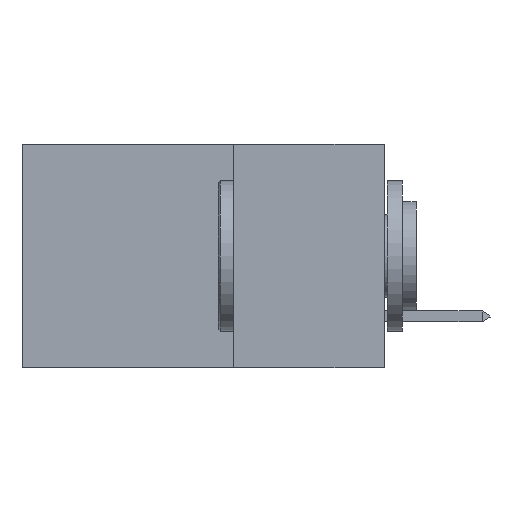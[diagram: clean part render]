
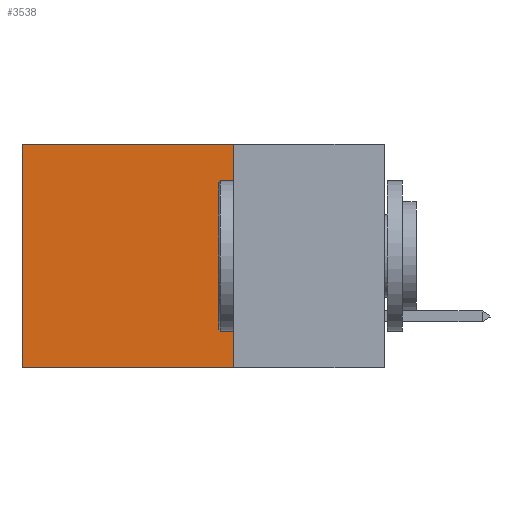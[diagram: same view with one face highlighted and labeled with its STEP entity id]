
A CAD part, left-side view. The second image highlights one B-rep face of the part: STEP entity #3538.
In plain terms, the highlighted planar face has unit normal (-1, 0, 0).
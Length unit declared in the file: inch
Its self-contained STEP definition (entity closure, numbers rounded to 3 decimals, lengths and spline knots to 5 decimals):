
#65 = DIRECTION ( 'NONE',  ( 0., 1., 0. ) ) ;
#426 = EDGE_CURVE ( 'NONE', #1089, #12628, #23306, .T. ) ;
#1089 = VERTEX_POINT ( 'NONE', #15708 ) ;
#2803 = EDGE_CURVE ( 'NONE', #9416, #12628, #25705, .T. ) ;
#3323 = AXIS2_PLACEMENT_3D ( 'NONE', #26052, #21626, #7824 ) ;
#3538 = ADVANCED_FACE ( 'NONE', ( #23547 ), #19427, .F. ) ;
#3616 = VERTEX_POINT ( 'NONE', #22016 ) ;
#6439 = DIRECTION ( 'NONE',  ( 0., 0., -1. ) ) ;
#7565 = CARTESIAN_POINT ( 'NONE',  ( 0.2875, 0.6, 0. ) ) ;
#7809 = LINE ( 'NONE', #16055, #29430 ) ;
#7824 = DIRECTION ( 'NONE',  ( 0., 0., -1. ) ) ;
#8056 = ORIENTED_EDGE ( 'NONE', *, *, #10873, .F. ) ;
#9325 = CARTESIAN_POINT ( 'NONE',  ( 0.2875, 0.6, 0. ) ) ;
#9416 = VERTEX_POINT ( 'NONE', #7565 ) ;
#10873 = EDGE_CURVE ( 'NONE', #3616, #1089, #7809, .T. ) ;
#11275 = DIRECTION ( 'NONE',  ( 0., 0., -1. ) ) ;
#12628 = VERTEX_POINT ( 'NONE', #18808 ) ;
#12774 = ORIENTED_EDGE ( 'NONE', *, *, #22019, .T. ) ;
#15352 = ORIENTED_EDGE ( 'NONE', *, *, #2803, .T. ) ;
#15708 = CARTESIAN_POINT ( 'NONE',  ( 0.2875, 0.25, -0.37 ) ) ;
#16055 = CARTESIAN_POINT ( 'NONE',  ( 0.2875, 0.25, 0. ) ) ;
#18363 = ORIENTED_EDGE ( 'NONE', *, *, #426, .F. ) ;
#18808 = CARTESIAN_POINT ( 'NONE',  ( 0.2875, 0.6, -0.37 ) ) ;
#19427 = PLANE ( 'NONE',  #3323 ) ;
#19621 = VECTOR ( 'NONE', #11275, 39.37008 ) ;
#21626 = DIRECTION ( 'NONE',  ( 1., 0., 0. ) ) ;
#21857 = VECTOR ( 'NONE', #65, 39.37008 ) ;
#22016 = CARTESIAN_POINT ( 'NONE',  ( 0.2875, 0.25, 0. ) ) ;
#22019 = EDGE_CURVE ( 'NONE', #3616, #9416, #28362, .T. ) ;
#23306 = LINE ( 'NONE', #25678, #21857 ) ;
#23547 = FACE_OUTER_BOUND ( 'NONE', #29643, .T. ) ;
#25453 = VECTOR ( 'NONE', #28675, 39.37008 ) ;
#25678 = CARTESIAN_POINT ( 'NONE',  ( 0.2875, 0.25, -0.37 ) ) ;
#25705 = LINE ( 'NONE', #9325, #19621 ) ;
#26052 = CARTESIAN_POINT ( 'NONE',  ( 0.2875, 0.25, 0. ) ) ;
#28362 = LINE ( 'NONE', #28767, #25453 ) ;
#28675 = DIRECTION ( 'NONE',  ( 0., 1., 0. ) ) ;
#28767 = CARTESIAN_POINT ( 'NONE',  ( 0.2875, 0.25, 0. ) ) ;
#29430 = VECTOR ( 'NONE', #6439, 39.37008 ) ;
#29643 = EDGE_LOOP ( 'NONE', ( #15352, #18363, #8056, #12774 ) ) ;
